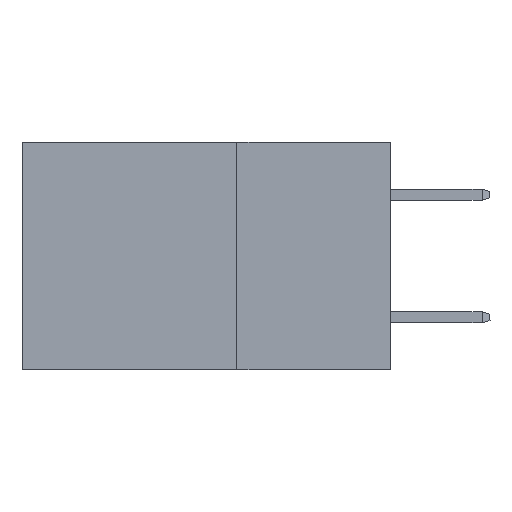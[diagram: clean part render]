
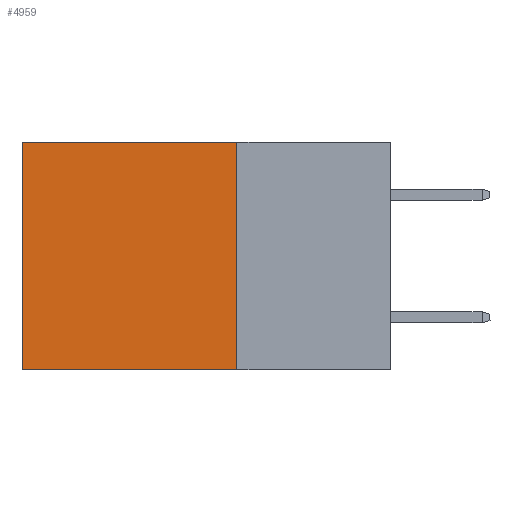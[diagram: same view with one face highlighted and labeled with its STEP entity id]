
A CAD part, left-side view. The second image highlights one B-rep face of the part: STEP entity #4959.
In plain terms, the highlighted planar face has unit normal (-1, 0, 0).
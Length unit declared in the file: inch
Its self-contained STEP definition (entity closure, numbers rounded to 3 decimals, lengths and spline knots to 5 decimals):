
#1063 = LINE ( 'NONE', #2463, #5305 ) ;
#1254 = PLANE ( 'NONE',  #11359 ) ;
#1339 = CARTESIAN_POINT ( 'NONE',  ( 0.2875, 0.25, 0. ) ) ;
#1641 = CARTESIAN_POINT ( 'NONE',  ( 0.2875, 0.25, -0.37 ) ) ;
#1667 = EDGE_CURVE ( 'NONE', #7823, #3002, #1063, .T. ) ;
#2463 = CARTESIAN_POINT ( 'NONE',  ( 0.2875, 0.25, 0. ) ) ;
#2469 = CARTESIAN_POINT ( 'NONE',  ( 0.2875, 0.6, -0.37 ) ) ;
#2543 = ORIENTED_EDGE ( 'NONE', *, *, #4057, .F. ) ;
#2592 = DIRECTION ( 'NONE',  ( 0., 1., 0. ) ) ;
#2721 = VECTOR ( 'NONE', #9865, 39.37008 ) ;
#2776 = VERTEX_POINT ( 'NONE', #5024 ) ;
#2877 = ORIENTED_EDGE ( 'NONE', *, *, #5756, .T. ) ;
#3002 = VERTEX_POINT ( 'NONE', #10013 ) ;
#3248 = DIRECTION ( 'NONE',  ( 0., 0., -1. ) ) ;
#3349 = LINE ( 'NONE', #1641, #9313 ) ;
#4057 = EDGE_CURVE ( 'NONE', #2776, #5616, #3349, .T. ) ;
#4509 = CARTESIAN_POINT ( 'NONE',  ( 0.2875, 0.25, 0. ) ) ;
#4959 = ADVANCED_FACE ( 'NONE', ( #6682 ), #1254, .F. ) ;
#5024 = CARTESIAN_POINT ( 'NONE',  ( 0.2875, 0.25, -0.37 ) ) ;
#5080 = DIRECTION ( 'NONE',  ( 1., 0., 0. ) ) ;
#5195 = LINE ( 'NONE', #10967, #2721 ) ;
#5222 = ORIENTED_EDGE ( 'NONE', *, *, #1667, .T. ) ;
#5296 = DIRECTION ( 'NONE',  ( 0., 0., -1. ) ) ;
#5305 = VECTOR ( 'NONE', #2592, 39.37008 ) ;
#5495 = VECTOR ( 'NONE', #5296, 39.37008 ) ;
#5616 = VERTEX_POINT ( 'NONE', #2469 ) ;
#5756 = EDGE_CURVE ( 'NONE', #3002, #5616, #10037, .T. ) ;
#6682 = FACE_OUTER_BOUND ( 'NONE', #9656, .T. ) ;
#7823 = VERTEX_POINT ( 'NONE', #4509 ) ;
#9313 = VECTOR ( 'NONE', #9369, 39.37008 ) ;
#9369 = DIRECTION ( 'NONE',  ( 0., 1., 0. ) ) ;
#9656 = EDGE_LOOP ( 'NONE', ( #2877, #2543, #9736, #5222 ) ) ;
#9736 = ORIENTED_EDGE ( 'NONE', *, *, #11030, .F. ) ;
#9865 = DIRECTION ( 'NONE',  ( 0., 0., -1. ) ) ;
#10013 = CARTESIAN_POINT ( 'NONE',  ( 0.2875, 0.6, 0. ) ) ;
#10037 = LINE ( 'NONE', #11719, #5495 ) ;
#10967 = CARTESIAN_POINT ( 'NONE',  ( 0.2875, 0.25, 0. ) ) ;
#11030 = EDGE_CURVE ( 'NONE', #7823, #2776, #5195, .T. ) ;
#11359 = AXIS2_PLACEMENT_3D ( 'NONE', #1339, #5080, #3248 ) ;
#11719 = CARTESIAN_POINT ( 'NONE',  ( 0.2875, 0.6, 0. ) ) ;
